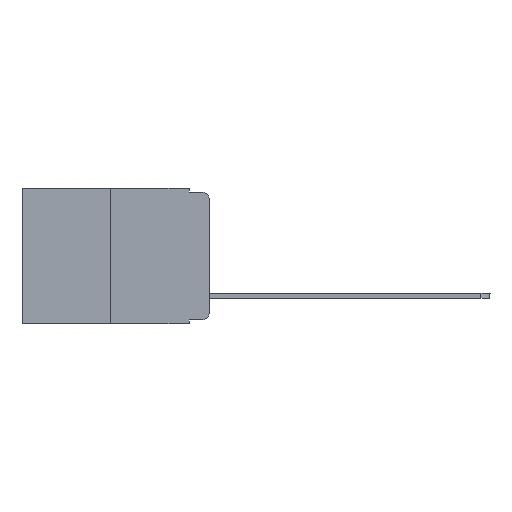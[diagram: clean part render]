
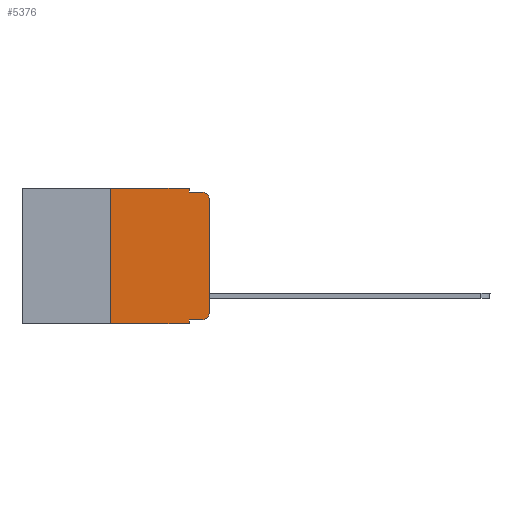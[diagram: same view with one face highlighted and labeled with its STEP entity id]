
A CAD part, left-side view. The second image highlights one B-rep face of the part: STEP entity #5376.
In plain terms, the highlighted planar face has unit normal (-1, 0, 0).
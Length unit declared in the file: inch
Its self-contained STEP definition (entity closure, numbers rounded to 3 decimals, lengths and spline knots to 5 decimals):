
#305 = VECTOR ( 'NONE', #2801, 39.37008 ) ;
#372 = CIRCLE ( 'NONE', #7971, 0.02 ) ;
#430 = VERTEX_POINT ( 'NONE', #5162 ) ;
#510 = VECTOR ( 'NONE', #859, 39.37008 ) ;
#559 = ORIENTED_EDGE ( 'NONE', *, *, #7701, .F. ) ;
#630 = LINE ( 'NONE', #4348, #3273 ) ;
#698 = CARTESIAN_POINT ( 'NONE',  ( 0., 0.25, 0. ) ) ;
#859 = DIRECTION ( 'NONE',  ( 0., 0., 1. ) ) ;
#1042 = PLANE ( 'NONE',  #4809 ) ;
#1193 = CIRCLE ( 'NONE', #8551, 0.02 ) ;
#1226 = FACE_OUTER_BOUND ( 'NONE', #10250, .T. ) ;
#1236 = VECTOR ( 'NONE', #9495, 39.37008 ) ;
#1442 = EDGE_CURVE ( 'NONE', #3952, #5267, #6116, .T. ) ;
#1445 = EDGE_CURVE ( 'NONE', #1737, #8536, #9280, .T. ) ;
#1737 = VERTEX_POINT ( 'NONE', #10903 ) ;
#1864 = DIRECTION ( 'NONE',  ( 1., 0., 0. ) ) ;
#2235 = DIRECTION ( 'NONE',  ( 0., 0., -1. ) ) ;
#2335 = ORIENTED_EDGE ( 'NONE', *, *, #11078, .T. ) ;
#2361 = ORIENTED_EDGE ( 'NONE', *, *, #7706, .F. ) ;
#2534 = DIRECTION ( 'NONE',  ( 0., 0., -1. ) ) ;
#2567 = LINE ( 'NONE', #698, #510 ) ;
#2736 = CARTESIAN_POINT ( 'NONE',  ( 0., 0.473, 0. ) ) ;
#2759 = ORIENTED_EDGE ( 'NONE', *, *, #10638, .F. ) ;
#2800 = CARTESIAN_POINT ( 'NONE',  ( 0., 0., 0. ) ) ;
#2801 = DIRECTION ( 'NONE',  ( 0., -1., 0. ) ) ;
#2974 = CARTESIAN_POINT ( 'NONE',  ( 0., 0.473, -0.343 ) ) ;
#3026 = CARTESIAN_POINT ( 'NONE',  ( 0., 0.02, -0.313 ) ) ;
#3273 = VECTOR ( 'NONE', #6176, 39.37008 ) ;
#3710 = CARTESIAN_POINT ( 'NONE',  ( 0., 0., -0.03 ) ) ;
#3738 = CARTESIAN_POINT ( 'NONE',  ( 0., 0.02, -0.333 ) ) ;
#3777 = ORIENTED_EDGE ( 'NONE', *, *, #1442, .F. ) ;
#3918 = DIRECTION ( 'NONE',  ( -1., 0., 0. ) ) ;
#3946 = ORIENTED_EDGE ( 'NONE', *, *, #4084, .F. ) ;
#3952 = VERTEX_POINT ( 'NONE', #9554 ) ;
#4013 = CARTESIAN_POINT ( 'NONE',  ( 0., 0.051, 0. ) ) ;
#4084 = EDGE_CURVE ( 'NONE', #5388, #6179, #8458, .T. ) ;
#4348 = CARTESIAN_POINT ( 'NONE',  ( 0., 0.051, 0. ) ) ;
#4809 = AXIS2_PLACEMENT_3D ( 'NONE', #2736, #1864, #7171 ) ;
#4932 = CARTESIAN_POINT ( 'NONE',  ( 0., 0.051, 0. ) ) ;
#5162 = CARTESIAN_POINT ( 'NONE',  ( 0., 0.051, -0.333 ) ) ;
#5267 = VERTEX_POINT ( 'NONE', #6990 ) ;
#5372 = ORIENTED_EDGE ( 'NONE', *, *, #1445, .T. ) ;
#5376 = ADVANCED_FACE ( 'NONE', ( #1226 ), #1042, .F. ) ;
#5388 = VERTEX_POINT ( 'NONE', #9799 ) ;
#5482 = EDGE_CURVE ( 'NONE', #11432, #10555, #10396, .T. ) ;
#5696 = DIRECTION ( 'NONE',  ( 0., 0., 1. ) ) ;
#6076 = ORIENTED_EDGE ( 'NONE', *, *, #7756, .T. ) ;
#6116 = LINE ( 'NONE', #11103, #1236 ) ;
#6176 = DIRECTION ( 'NONE',  ( 0., 0., -1. ) ) ;
#6179 = VERTEX_POINT ( 'NONE', #4932 ) ;
#6990 = CARTESIAN_POINT ( 'NONE',  ( 0., 0.02, -0.01 ) ) ;
#7171 = DIRECTION ( 'NONE',  ( 0., 0., -1. ) ) ;
#7485 = LINE ( 'NONE', #9655, #11083 ) ;
#7508 = EDGE_CURVE ( 'NONE', #8523, #1737, #372, .T. ) ;
#7701 = EDGE_CURVE ( 'NONE', #6179, #3952, #630, .T. ) ;
#7706 = EDGE_CURVE ( 'NONE', #11432, #5388, #2567, .T. ) ;
#7756 = EDGE_CURVE ( 'NONE', #8536, #5267, #1193, .T. ) ;
#7971 = AXIS2_PLACEMENT_3D ( 'NONE', #3026, #3918, #11006 ) ;
#8019 = DIRECTION ( 'NONE',  ( 0., -1., 0. ) ) ;
#8458 = LINE ( 'NONE', #10684, #305 ) ;
#8523 = VERTEX_POINT ( 'NONE', #3738 ) ;
#8536 = VERTEX_POINT ( 'NONE', #3710 ) ;
#8551 = AXIS2_PLACEMENT_3D ( 'NONE', #11424, #9620, #2534 ) ;
#8571 = LINE ( 'NONE', #4013, #9136 ) ;
#8761 = CARTESIAN_POINT ( 'NONE',  ( 0., 0.051, -0.343 ) ) ;
#9001 = VECTOR ( 'NONE', #11018, 39.37008 ) ;
#9136 = VECTOR ( 'NONE', #2235, 39.37008 ) ;
#9213 = CARTESIAN_POINT ( 'NONE',  ( 0., 0.25, -0.343 ) ) ;
#9280 = LINE ( 'NONE', #2800, #10694 ) ;
#9301 = ORIENTED_EDGE ( 'NONE', *, *, #5482, .T. ) ;
#9495 = DIRECTION ( 'NONE',  ( 0., -1., 0. ) ) ;
#9554 = CARTESIAN_POINT ( 'NONE',  ( 0., 0.051, -0.01 ) ) ;
#9620 = DIRECTION ( 'NONE',  ( -1., 0., 0. ) ) ;
#9655 = CARTESIAN_POINT ( 'NONE',  ( 0., 0.051, -0.333 ) ) ;
#9799 = CARTESIAN_POINT ( 'NONE',  ( 0., 0.25, 0. ) ) ;
#10250 = EDGE_LOOP ( 'NONE', ( #5372, #6076, #3777, #559, #3946, #2361, #9301, #2759, #2335, #11473 ) ) ;
#10396 = LINE ( 'NONE', #2974, #9001 ) ;
#10555 = VERTEX_POINT ( 'NONE', #8761 ) ;
#10638 = EDGE_CURVE ( 'NONE', #430, #10555, #8571, .T. ) ;
#10684 = CARTESIAN_POINT ( 'NONE',  ( 0., 0.473, 0. ) ) ;
#10694 = VECTOR ( 'NONE', #5696, 39.37008 ) ;
#10903 = CARTESIAN_POINT ( 'NONE',  ( 0., 0., -0.313 ) ) ;
#11006 = DIRECTION ( 'NONE',  ( 0., 0., -1. ) ) ;
#11018 = DIRECTION ( 'NONE',  ( 0., -1., 0. ) ) ;
#11078 = EDGE_CURVE ( 'NONE', #430, #8523, #7485, .T. ) ;
#11083 = VECTOR ( 'NONE', #8019, 39.37008 ) ;
#11103 = CARTESIAN_POINT ( 'NONE',  ( 0., 0.051, -0.01 ) ) ;
#11424 = CARTESIAN_POINT ( 'NONE',  ( 0., 0.02, -0.03 ) ) ;
#11432 = VERTEX_POINT ( 'NONE', #9213 ) ;
#11473 = ORIENTED_EDGE ( 'NONE', *, *, #7508, .T. ) ;
